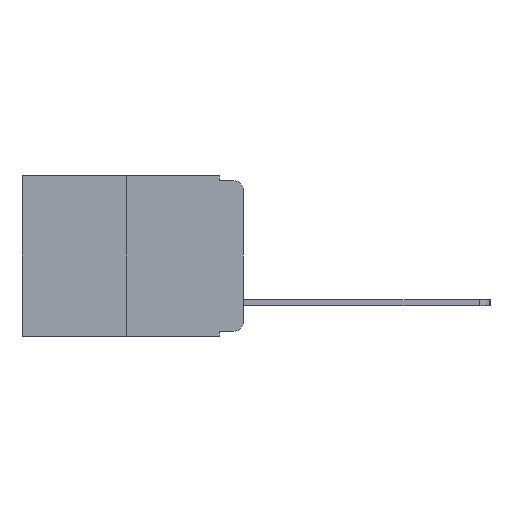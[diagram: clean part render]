
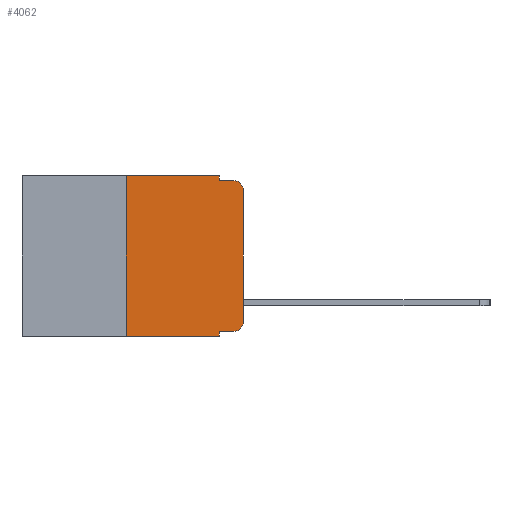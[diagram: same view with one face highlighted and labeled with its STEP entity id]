
A CAD part, left-side view. The second image highlights one B-rep face of the part: STEP entity #4062.
In plain terms, the highlighted planar face has unit normal (-1, 0, 0).
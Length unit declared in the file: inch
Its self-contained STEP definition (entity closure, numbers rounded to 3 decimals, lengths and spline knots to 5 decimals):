
#376 = AXIS2_PLACEMENT_3D ( 'NONE', #9890, #21528, #11573 ) ;
#430 = DIRECTION ( 'NONE',  ( 0., 0., -1. ) ) ;
#1140 = ORIENTED_EDGE ( 'NONE', *, *, #16648, .T. ) ;
#1295 = CARTESIAN_POINT ( 'NONE',  ( 0., 0.473, 0. ) ) ;
#1390 = DIRECTION ( 'NONE',  ( 0., 0., 1. ) ) ;
#3051 = VERTEX_POINT ( 'NONE', #20355 ) ;
#3240 = DIRECTION ( 'NONE',  ( 0., -1., 0. ) ) ;
#3381 = VERTEX_POINT ( 'NONE', #13061 ) ;
#3646 = DIRECTION ( 'NONE',  ( -1., 0., 0. ) ) ;
#4062 = ADVANCED_FACE ( 'NONE', ( #4647 ), #17590, .F. ) ;
#4451 = CARTESIAN_POINT ( 'NONE',  ( 0., 0.25, 0. ) ) ;
#4517 = CARTESIAN_POINT ( 'NONE',  ( 0., 0.473, -0.343 ) ) ;
#4647 = FACE_OUTER_BOUND ( 'NONE', #19963, .T. ) ;
#4731 = VECTOR ( 'NONE', #430, 39.37008 ) ;
#4962 = ORIENTED_EDGE ( 'NONE', *, *, #12176, .F. ) ;
#5090 = CARTESIAN_POINT ( 'NONE',  ( 0., 0.051, -0.01 ) ) ;
#5370 = LINE ( 'NONE', #16449, #9577 ) ;
#5466 = LINE ( 'NONE', #4517, #14167 ) ;
#5847 = LINE ( 'NONE', #21265, #4731 ) ;
#6306 = DIRECTION ( 'NONE',  ( 0., -1., 0. ) ) ;
#6352 = VERTEX_POINT ( 'NONE', #14029 ) ;
#6655 = DIRECTION ( 'NONE',  ( 0., -1., 0. ) ) ;
#6892 = CARTESIAN_POINT ( 'NONE',  ( 0., 0.473, 0. ) ) ;
#7373 = DIRECTION ( 'NONE',  ( 1., 0., 0. ) ) ;
#7525 = EDGE_CURVE ( 'NONE', #20130, #18553, #20919, .T. ) ;
#7581 = VECTOR ( 'NONE', #14587, 39.37008 ) ;
#7837 = EDGE_CURVE ( 'NONE', #12913, #14687, #5466, .T. ) ;
#7856 = AXIS2_PLACEMENT_3D ( 'NONE', #14131, #3646, #15809 ) ;
#8036 = ORIENTED_EDGE ( 'NONE', *, *, #21658, .F. ) ;
#8141 = LINE ( 'NONE', #12912, #7581 ) ;
#8416 = CARTESIAN_POINT ( 'NONE',  ( 0., 0., -0.313 ) ) ;
#8624 = VERTEX_POINT ( 'NONE', #18611 ) ;
#8736 = EDGE_CURVE ( 'NONE', #6352, #20130, #17730, .T. ) ;
#8775 = VERTEX_POINT ( 'NONE', #10676 ) ;
#8900 = LINE ( 'NONE', #5090, #21729 ) ;
#9007 = CARTESIAN_POINT ( 'NONE',  ( 0., 0.051, -0.333 ) ) ;
#9172 = ORIENTED_EDGE ( 'NONE', *, *, #13310, .F. ) ;
#9577 = VECTOR ( 'NONE', #18109, 39.37008 ) ;
#9890 = CARTESIAN_POINT ( 'NONE',  ( 0., 0.02, -0.03 ) ) ;
#9935 = EDGE_CURVE ( 'NONE', #6352, #14687, #8141, .T. ) ;
#10676 = CARTESIAN_POINT ( 'NONE',  ( 0., 0., -0.03 ) ) ;
#11050 = EDGE_CURVE ( 'NONE', #12913, #13660, #22300, .T. ) ;
#11572 = ORIENTED_EDGE ( 'NONE', *, *, #7525, .T. ) ;
#11573 = DIRECTION ( 'NONE',  ( 0., 0., -1. ) ) ;
#12176 = EDGE_CURVE ( 'NONE', #3051, #3381, #5847, .T. ) ;
#12912 = CARTESIAN_POINT ( 'NONE',  ( 0., 0.051, 0. ) ) ;
#12913 = VERTEX_POINT ( 'NONE', #17902 ) ;
#13061 = CARTESIAN_POINT ( 'NONE',  ( 0., 0.051, -0.01 ) ) ;
#13310 = EDGE_CURVE ( 'NONE', #3381, #8624, #8900, .T. ) ;
#13316 = VECTOR ( 'NONE', #20737, 39.37008 ) ;
#13478 = CARTESIAN_POINT ( 'NONE',  ( 0., 0.051, -0.343 ) ) ;
#13660 = VERTEX_POINT ( 'NONE', #4451 ) ;
#14029 = CARTESIAN_POINT ( 'NONE',  ( 0., 0.051, -0.333 ) ) ;
#14131 = CARTESIAN_POINT ( 'NONE',  ( 0., 0.02, -0.313 ) ) ;
#14167 = VECTOR ( 'NONE', #6306, 39.37008 ) ;
#14220 = ORIENTED_EDGE ( 'NONE', *, *, #17754, .T. ) ;
#14587 = DIRECTION ( 'NONE',  ( 0., 0., -1. ) ) ;
#14687 = VERTEX_POINT ( 'NONE', #13478 ) ;
#14970 = ORIENTED_EDGE ( 'NONE', *, *, #8736, .T. ) ;
#15809 = DIRECTION ( 'NONE',  ( 0., 0., -1. ) ) ;
#16025 = ORIENTED_EDGE ( 'NONE', *, *, #7837, .T. ) ;
#16449 = CARTESIAN_POINT ( 'NONE',  ( 0., 0., 0. ) ) ;
#16648 = EDGE_CURVE ( 'NONE', #8775, #8624, #16924, .T. ) ;
#16706 = LINE ( 'NONE', #1295, #21122 ) ;
#16924 = CIRCLE ( 'NONE', #376, 0.02 ) ;
#17030 = CARTESIAN_POINT ( 'NONE',  ( 0., 0.25, 0. ) ) ;
#17590 = PLANE ( 'NONE',  #20083 ) ;
#17730 = LINE ( 'NONE', #9007, #13316 ) ;
#17754 = EDGE_CURVE ( 'NONE', #18553, #8775, #5370, .T. ) ;
#17875 = VECTOR ( 'NONE', #1390, 39.37008 ) ;
#17898 = DIRECTION ( 'NONE',  ( 0., 0., -1. ) ) ;
#17902 = CARTESIAN_POINT ( 'NONE',  ( 0., 0.25, -0.343 ) ) ;
#18109 = DIRECTION ( 'NONE',  ( 0., 0., 1. ) ) ;
#18553 = VERTEX_POINT ( 'NONE', #8416 ) ;
#18611 = CARTESIAN_POINT ( 'NONE',  ( 0., 0.02, -0.01 ) ) ;
#19963 = EDGE_LOOP ( 'NONE', ( #14220, #1140, #9172, #4962, #8036, #21464, #16025, #20425, #14970, #11572 ) ) ;
#20083 = AXIS2_PLACEMENT_3D ( 'NONE', #6892, #7373, #17898 ) ;
#20130 = VERTEX_POINT ( 'NONE', #21995 ) ;
#20355 = CARTESIAN_POINT ( 'NONE',  ( 0., 0.051, 0. ) ) ;
#20425 = ORIENTED_EDGE ( 'NONE', *, *, #9935, .F. ) ;
#20737 = DIRECTION ( 'NONE',  ( 0., -1., 0. ) ) ;
#20919 = CIRCLE ( 'NONE', #7856, 0.02 ) ;
#21122 = VECTOR ( 'NONE', #3240, 39.37008 ) ;
#21265 = CARTESIAN_POINT ( 'NONE',  ( 0., 0.051, 0. ) ) ;
#21464 = ORIENTED_EDGE ( 'NONE', *, *, #11050, .F. ) ;
#21528 = DIRECTION ( 'NONE',  ( -1., 0., 0. ) ) ;
#21658 = EDGE_CURVE ( 'NONE', #13660, #3051, #16706, .T. ) ;
#21729 = VECTOR ( 'NONE', #6655, 39.37008 ) ;
#21995 = CARTESIAN_POINT ( 'NONE',  ( 0., 0.02, -0.333 ) ) ;
#22300 = LINE ( 'NONE', #17030, #17875 ) ;
